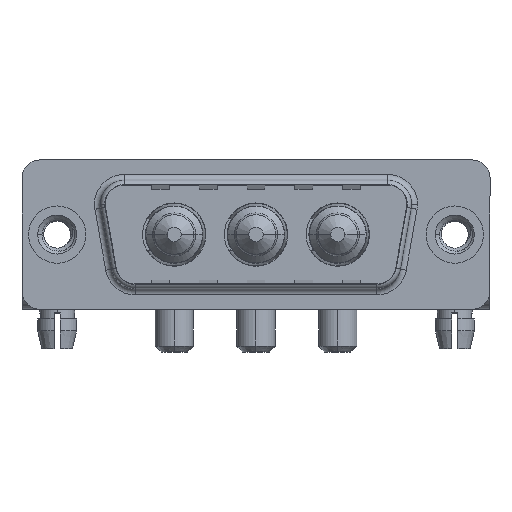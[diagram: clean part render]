
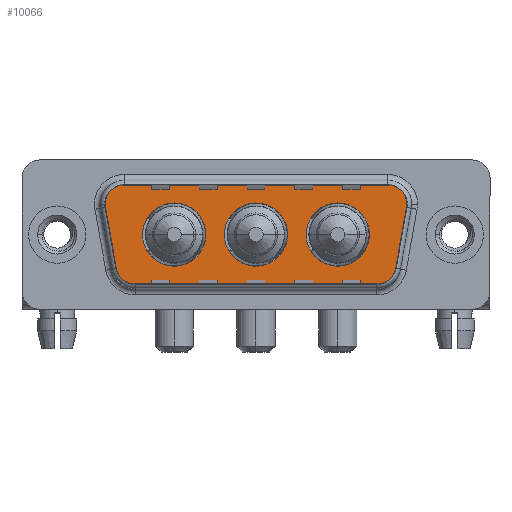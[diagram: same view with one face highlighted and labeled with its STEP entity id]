
A CAD part, top view. The second image highlights one B-rep face of the part: STEP entity #10066.
In plain terms, the highlighted planar face has unit normal (0, 0, 1).
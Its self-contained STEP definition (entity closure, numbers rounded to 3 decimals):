
#252 = CARTESIAN_POINT ( 'NONE',  ( 29.859, 2.553, 0. ) ) ;
#299 = VERTEX_POINT ( 'NONE', #8612 ) ;
#306 = CIRCLE ( 'NONE', #10531, 2.65 ) ;
#466 = ORIENTED_EDGE ( 'NONE', *, *, #11831, .T. ) ;
#607 = ORIENTED_EDGE ( 'NONE', *, *, #7899, .F. ) ;
#733 = AXIS2_PLACEMENT_3D ( 'NONE', #7809, #4208, #7581 ) ;
#1183 = DIRECTION ( 'NONE',  ( 1., 0., 0. ) ) ;
#1257 = EDGE_CURVE ( 'NONE', #2389, #299, #11185, .T. ) ;
#1343 = DIRECTION ( 'NONE',  ( 0.174, -0.985, 0. ) ) ;
#1386 = CARTESIAN_POINT ( 'NONE',  ( 27.889, 4.9, 0. ) ) ;
#1409 = AXIS2_PLACEMENT_3D ( 'NONE', #10096, #5256, #14867 ) ;
#1602 = VERTEX_POINT ( 'NONE', #2742 ) ;
#1804 = VERTEX_POINT ( 'NONE', #5297 ) ;
#1851 = AXIS2_PLACEMENT_3D ( 'NONE', #11071, #4962, #12165 ) ;
#1858 = CARTESIAN_POINT ( 'NONE',  ( 6.434, -4.9, 0. ) ) ;
#2148 = DIRECTION ( 'NONE',  ( -1., 0., 0. ) ) ;
#2169 = VERTEX_POINT ( 'NONE', #1386 ) ;
#2389 = VERTEX_POINT ( 'NONE', #1858 ) ;
#2390 = FACE_OUTER_BOUND ( 'NONE', #11779, .T. ) ;
#2515 = VECTOR ( 'NONE', #9313, 1000. ) ;
#2579 = DIRECTION ( 'NONE',  ( 1., 0., 0. ) ) ;
#2675 = DIRECTION ( 'NONE',  ( 0., 0., 1. ) ) ;
#2742 = CARTESIAN_POINT ( 'NONE',  ( 29.889, 2.9, 0. ) ) ;
#2827 = LINE ( 'NONE', #13225, #15414 ) ;
#2883 = EDGE_CURVE ( 'NONE', #8850, #2389, #3260, .T. ) ;
#2934 = VECTOR ( 'NONE', #7597, 1000. ) ;
#3019 = CIRCLE ( 'NONE', #733, 2. ) ;
#3208 = EDGE_CURVE ( 'NONE', #14292, #13740, #3019, .T. ) ;
#3241 = PLANE ( 'NONE',  #10915 ) ;
#3260 = CIRCLE ( 'NONE', #12004, 2. ) ;
#3434 = EDGE_CURVE ( 'NONE', #8265, #10778, #10208, .T. ) ;
#3457 = CARTESIAN_POINT ( 'NONE',  ( 12.45, 0., 0. ) ) ;
#3844 = DIRECTION ( 'NONE',  ( 0., 0., 1. ) ) ;
#4000 = ORIENTED_EDGE ( 'NONE', *, *, #1257, .T. ) ;
#4160 = ORIENTED_EDGE ( 'NONE', *, *, #4364, .F. ) ;
#4198 = ORIENTED_EDGE ( 'NONE', *, *, #14427, .T. ) ;
#4208 = DIRECTION ( 'NONE',  ( 0., 0., 1. ) ) ;
#4259 = ORIENTED_EDGE ( 'NONE', *, *, #2883, .T. ) ;
#4364 = EDGE_CURVE ( 'NONE', #4424, #14441, #8497, .T. ) ;
#4424 = VERTEX_POINT ( 'NONE', #10268 ) ;
#4661 = DIRECTION ( 'NONE',  ( 1., 0., 0. ) ) ;
#4667 = CARTESIAN_POINT ( 'NONE',  ( 16.65, 0., 0. ) ) ;
#4789 = CARTESIAN_POINT ( 'NONE',  ( 4.464, -3.247, 0. ) ) ;
#4962 = DIRECTION ( 'NONE',  ( 0., 0., 1. ) ) ;
#5118 = VERTEX_POINT ( 'NONE', #12301 ) ;
#5256 = DIRECTION ( 'NONE',  ( 0., 0., 1. ) ) ;
#5297 = CARTESIAN_POINT ( 'NONE',  ( 20.85, 0., 0. ) ) ;
#5636 = DIRECTION ( 'NONE',  ( 1., 0., 0. ) ) ;
#5694 = DIRECTION ( 'NONE',  ( 0., 0., 1. ) ) ;
#5719 = VERTEX_POINT ( 'NONE', #252 ) ;
#5725 = FACE_BOUND ( 'NONE', #13720, .T. ) ;
#5964 = AXIS2_PLACEMENT_3D ( 'NONE', #10536, #12734, #4661 ) ;
#6050 = CARTESIAN_POINT ( 'NONE',  ( 29.859, 2.553, 0. ) ) ;
#6058 = ORIENTED_EDGE ( 'NONE', *, *, #13101, .F. ) ;
#6182 = CIRCLE ( 'NONE', #7456, 2.65 ) ;
#6201 = DIRECTION ( 'NONE',  ( 0.174, 0.985, 0. ) ) ;
#6242 = DIRECTION ( 'NONE',  ( 1., 0., 0. ) ) ;
#6437 = ORIENTED_EDGE ( 'NONE', *, *, #3208, .T. ) ;
#6683 = EDGE_LOOP ( 'NONE', ( #6058, #12113 ) ) ;
#6708 = CARTESIAN_POINT ( 'NONE',  ( 6.434, -4.9, 0. ) ) ;
#6735 = CARTESIAN_POINT ( 'NONE',  ( 9.8, 0., 0. ) ) ;
#7043 = CARTESIAN_POINT ( 'NONE',  ( 19.3, 0., 0. ) ) ;
#7129 = CARTESIAN_POINT ( 'NONE',  ( 26.866, -2.9, 0. ) ) ;
#7278 = CARTESIAN_POINT ( 'NONE',  ( 5.411, 4.9, 0. ) ) ;
#7322 = VERTEX_POINT ( 'NONE', #8251 ) ;
#7405 = CIRCLE ( 'NONE', #9904, 2. ) ;
#7456 = AXIS2_PLACEMENT_3D ( 'NONE', #10093, #8370, #1183 ) ;
#7514 = ORIENTED_EDGE ( 'NONE', *, *, #12892, .F. ) ;
#7581 = DIRECTION ( 'NONE',  ( 1., 0., 0. ) ) ;
#7597 = DIRECTION ( 'NONE',  ( 1., 0., 0. ) ) ;
#7704 = CIRCLE ( 'NONE', #9952, 2.65 ) ;
#7752 = AXIS2_PLACEMENT_3D ( 'NONE', #6735, #7849, #5636 ) ;
#7809 = CARTESIAN_POINT ( 'NONE',  ( 5.411, 2.9, 0. ) ) ;
#7849 = DIRECTION ( 'NONE',  ( 0., 0., 1. ) ) ;
#7877 = CARTESIAN_POINT ( 'NONE',  ( 3.441, 2.553, 0. ) ) ;
#7899 = EDGE_CURVE ( 'NONE', #10778, #8265, #306, .T. ) ;
#7980 = VECTOR ( 'NONE', #6201, 1000. ) ;
#8251 = CARTESIAN_POINT ( 'NONE',  ( 28.836, -3.247, 0. ) ) ;
#8265 = VERTEX_POINT ( 'NONE', #11852 ) ;
#8316 = FACE_BOUND ( 'NONE', #6683, .T. ) ;
#8319 = ORIENTED_EDGE ( 'NONE', *, *, #14107, .T. ) ;
#8370 = DIRECTION ( 'NONE',  ( 0., 0., 1. ) ) ;
#8497 = CIRCLE ( 'NONE', #7752, 2.65 ) ;
#8577 = CIRCLE ( 'NONE', #1851, 2. ) ;
#8612 = CARTESIAN_POINT ( 'NONE',  ( 26.866, -4.9, 0. ) ) ;
#8850 = VERTEX_POINT ( 'NONE', #4789 ) ;
#8862 = ORIENTED_EDGE ( 'NONE', *, *, #11173, .T. ) ;
#9175 = FACE_BOUND ( 'NONE', #10854, .T. ) ;
#9313 = DIRECTION ( 'NONE',  ( -1., 0., 0. ) ) ;
#9469 = LINE ( 'NONE', #7278, #2515 ) ;
#9667 = EDGE_CURVE ( 'NONE', #1602, #2169, #8577, .T. ) ;
#9904 = AXIS2_PLACEMENT_3D ( 'NONE', #14167, #12856, #2148 ) ;
#9952 = AXIS2_PLACEMENT_3D ( 'NONE', #10949, #3844, #10872 ) ;
#10066 = ADVANCED_FACE ( 'NONE', ( #9175, #8316, #5725, #2390 ), #3241, .T. ) ;
#10093 = CARTESIAN_POINT ( 'NONE',  ( 9.8, 0., 0. ) ) ;
#10096 = CARTESIAN_POINT ( 'NONE',  ( 23.5, 0., 0. ) ) ;
#10148 = ORIENTED_EDGE ( 'NONE', *, *, #3434, .F. ) ;
#10208 = CIRCLE ( 'NONE', #5964, 2.65 ) ;
#10268 = CARTESIAN_POINT ( 'NONE',  ( 7.15, 0., 0. ) ) ;
#10504 = DIRECTION ( 'NONE',  ( 1., 0., 0. ) ) ;
#10531 = AXIS2_PLACEMENT_3D ( 'NONE', #4667, #13517, #2579 ) ;
#10536 = CARTESIAN_POINT ( 'NONE',  ( 16.65, 0., 0. ) ) ;
#10615 = EDGE_CURVE ( 'NONE', #1804, #5118, #14876, .T. ) ;
#10737 = ORIENTED_EDGE ( 'NONE', *, *, #9667, .T. ) ;
#10778 = VERTEX_POINT ( 'NONE', #7043 ) ;
#10854 = EDGE_LOOP ( 'NONE', ( #607, #10148 ) ) ;
#10872 = DIRECTION ( 'NONE',  ( 1., 0., 0. ) ) ;
#10915 = AXIS2_PLACEMENT_3D ( 'NONE', #7129, #12785, #10504 ) ;
#10949 = CARTESIAN_POINT ( 'NONE',  ( 23.5, 0., 0. ) ) ;
#11071 = CARTESIAN_POINT ( 'NONE',  ( 27.889, 2.9, 0. ) ) ;
#11173 = EDGE_CURVE ( 'NONE', #5719, #1602, #7405, .T. ) ;
#11185 = LINE ( 'NONE', #6708, #2934 ) ;
#11779 = EDGE_LOOP ( 'NONE', ( #15122, #8319, #8862, #10737, #4198, #6437, #466, #4259, #4000 ) ) ;
#11831 = EDGE_CURVE ( 'NONE', #13740, #8850, #2827, .T. ) ;
#11852 = CARTESIAN_POINT ( 'NONE',  ( 14., 0., 0. ) ) ;
#11886 = CARTESIAN_POINT ( 'NONE',  ( 6.434, -2.9, 0. ) ) ;
#12004 = AXIS2_PLACEMENT_3D ( 'NONE', #11886, #5694, #15389 ) ;
#12025 = LINE ( 'NONE', #6050, #7980 ) ;
#12063 = CARTESIAN_POINT ( 'NONE',  ( 26.866, -2.9, 0. ) ) ;
#12113 = ORIENTED_EDGE ( 'NONE', *, *, #10615, .F. ) ;
#12165 = DIRECTION ( 'NONE',  ( -1., 0., 0. ) ) ;
#12301 = CARTESIAN_POINT ( 'NONE',  ( 26.15, 0., 0. ) ) ;
#12734 = DIRECTION ( 'NONE',  ( 0., 0., 1. ) ) ;
#12785 = DIRECTION ( 'NONE',  ( 0., 0., 1. ) ) ;
#12856 = DIRECTION ( 'NONE',  ( 0., 0., 1. ) ) ;
#12892 = EDGE_CURVE ( 'NONE', #14441, #4424, #6182, .T. ) ;
#13033 = EDGE_CURVE ( 'NONE', #299, #7322, #13459, .T. ) ;
#13101 = EDGE_CURVE ( 'NONE', #5118, #1804, #7704, .T. ) ;
#13225 = CARTESIAN_POINT ( 'NONE',  ( 3.441, 2.553, 0. ) ) ;
#13459 = CIRCLE ( 'NONE', #14690, 2. ) ;
#13517 = DIRECTION ( 'NONE',  ( 0., 0., 1. ) ) ;
#13720 = EDGE_LOOP ( 'NONE', ( #7514, #4160 ) ) ;
#13740 = VERTEX_POINT ( 'NONE', #7877 ) ;
#14107 = EDGE_CURVE ( 'NONE', #7322, #5719, #12025, .T. ) ;
#14167 = CARTESIAN_POINT ( 'NONE',  ( 27.889, 2.9, 0. ) ) ;
#14292 = VERTEX_POINT ( 'NONE', #15032 ) ;
#14427 = EDGE_CURVE ( 'NONE', #2169, #14292, #9469, .T. ) ;
#14441 = VERTEX_POINT ( 'NONE', #3457 ) ;
#14690 = AXIS2_PLACEMENT_3D ( 'NONE', #12063, #2675, #6242 ) ;
#14867 = DIRECTION ( 'NONE',  ( 1., 0., 0. ) ) ;
#14876 = CIRCLE ( 'NONE', #1409, 2.65 ) ;
#15032 = CARTESIAN_POINT ( 'NONE',  ( 5.411, 4.9, 0. ) ) ;
#15122 = ORIENTED_EDGE ( 'NONE', *, *, #13033, .T. ) ;
#15389 = DIRECTION ( 'NONE',  ( -1., 0., 0. ) ) ;
#15414 = VECTOR ( 'NONE', #1343, 1000. ) ;
